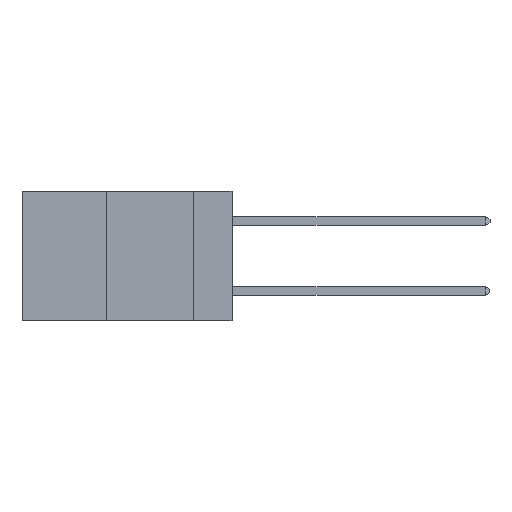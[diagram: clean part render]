
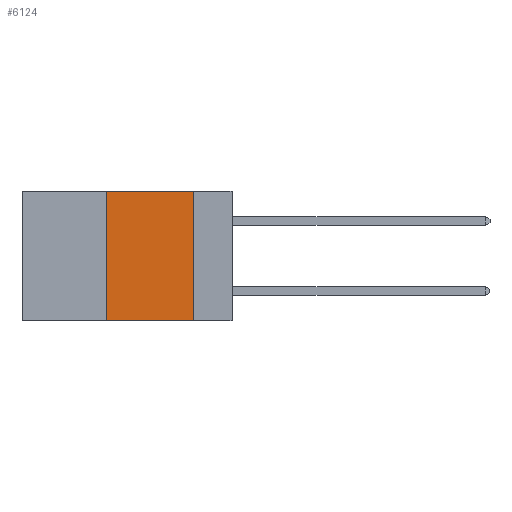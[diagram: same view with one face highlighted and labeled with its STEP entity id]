
A CAD part, left-side view. The second image highlights one B-rep face of the part: STEP entity #6124.
In plain terms, the highlighted planar face has unit normal (-1, 0, 0).
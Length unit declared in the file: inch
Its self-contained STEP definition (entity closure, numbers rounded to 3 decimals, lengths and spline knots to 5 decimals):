
#845 = LINE ( 'NONE', #10905, #8267 ) ;
#1444 = CARTESIAN_POINT ( 'NONE',  ( 0., 0.36, 0. ) ) ;
#1905 = DIRECTION ( 'NONE',  ( 0., 0., 1. ) ) ;
#2481 = DIRECTION ( 'NONE',  ( 0., -1., 0. ) ) ;
#2591 = CARTESIAN_POINT ( 'NONE',  ( 0., 0.6, -0.37 ) ) ;
#3292 = LINE ( 'NONE', #13190, #18359 ) ;
#3819 = VERTEX_POINT ( 'NONE', #10827 ) ;
#5155 = AXIS2_PLACEMENT_3D ( 'NONE', #9722, #6708, #16998 ) ;
#5396 = CARTESIAN_POINT ( 'NONE',  ( 0., 0.6, 0. ) ) ;
#5522 = ORIENTED_EDGE ( 'NONE', *, *, #16718, .F. ) ;
#5979 = EDGE_CURVE ( 'NONE', #3819, #15244, #3292, .T. ) ;
#6124 = ADVANCED_FACE ( 'NONE', ( #12452 ), #15613, .F. ) ;
#6213 = ORIENTED_EDGE ( 'NONE', *, *, #5979, .F. ) ;
#6708 = DIRECTION ( 'NONE',  ( 1., 0., 0. ) ) ;
#6790 = ORIENTED_EDGE ( 'NONE', *, *, #10926, .F. ) ;
#7905 = VECTOR ( 'NONE', #13115, 39.37008 ) ;
#8166 = ORIENTED_EDGE ( 'NONE', *, *, #18272, .T. ) ;
#8267 = VECTOR ( 'NONE', #1905, 39.37008 ) ;
#9722 = CARTESIAN_POINT ( 'NONE',  ( 0., 0.6, 0. ) ) ;
#9756 = VERTEX_POINT ( 'NONE', #16144 ) ;
#10626 = DIRECTION ( 'NONE',  ( 0., 0., -1. ) ) ;
#10827 = CARTESIAN_POINT ( 'NONE',  ( 0., 0.11, 0. ) ) ;
#10905 = CARTESIAN_POINT ( 'NONE',  ( 0., 0.36, 0. ) ) ;
#10926 = EDGE_CURVE ( 'NONE', #15119, #3819, #13878, .T. ) ;
#12452 = FACE_OUTER_BOUND ( 'NONE', #17790, .T. ) ;
#13115 = DIRECTION ( 'NONE',  ( 0., -1., 0. ) ) ;
#13190 = CARTESIAN_POINT ( 'NONE',  ( 0., 0.11, 0. ) ) ;
#13878 = LINE ( 'NONE', #5396, #17144 ) ;
#15119 = VERTEX_POINT ( 'NONE', #1444 ) ;
#15244 = VERTEX_POINT ( 'NONE', #18678 ) ;
#15613 = PLANE ( 'NONE',  #5155 ) ;
#15760 = LINE ( 'NONE', #2591, #7905 ) ;
#16144 = CARTESIAN_POINT ( 'NONE',  ( 0., 0.36, -0.37 ) ) ;
#16718 = EDGE_CURVE ( 'NONE', #9756, #15119, #845, .T. ) ;
#16998 = DIRECTION ( 'NONE',  ( 0., 0., -1. ) ) ;
#17144 = VECTOR ( 'NONE', #2481, 39.37008 ) ;
#17790 = EDGE_LOOP ( 'NONE', ( #6213, #6790, #5522, #8166 ) ) ;
#18272 = EDGE_CURVE ( 'NONE', #9756, #15244, #15760, .T. ) ;
#18359 = VECTOR ( 'NONE', #10626, 39.37008 ) ;
#18678 = CARTESIAN_POINT ( 'NONE',  ( 0., 0.11, -0.37 ) ) ;
